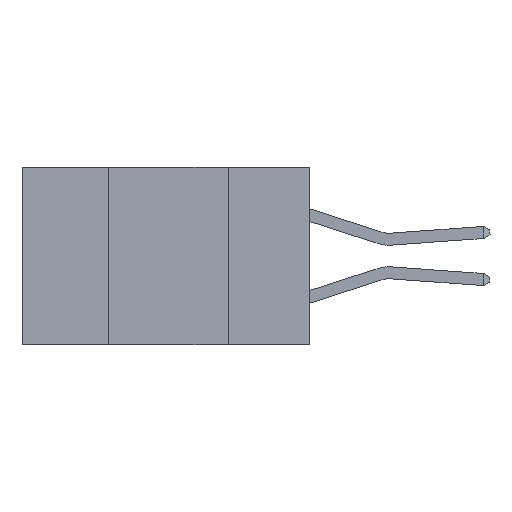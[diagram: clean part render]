
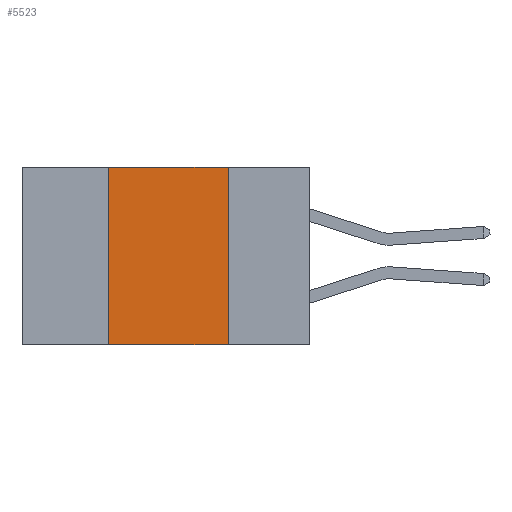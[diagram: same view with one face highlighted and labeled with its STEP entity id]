
A CAD part, left-side view. The second image highlights one B-rep face of the part: STEP entity #5523.
In plain terms, the highlighted planar face has unit normal (-1, 0, 0).
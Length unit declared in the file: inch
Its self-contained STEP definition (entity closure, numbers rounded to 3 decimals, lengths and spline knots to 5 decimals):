
#82 = FACE_OUTER_BOUND ( 'NONE', #3241, .T. ) ;
#1357 = ORIENTED_EDGE ( 'NONE', *, *, #4024, .F. ) ;
#2063 = CARTESIAN_POINT ( 'NONE',  ( 0., 0.6, -0.37 ) ) ;
#3241 = EDGE_LOOP ( 'NONE', ( #1357, #10445, #5084, #19178 ) ) ;
#3884 = DIRECTION ( 'NONE',  ( 0., -1., 0. ) ) ;
#4024 = EDGE_CURVE ( 'NONE', #11356, #23159, #18539, .T. ) ;
#4335 = LINE ( 'NONE', #2063, #17885 ) ;
#5084 = ORIENTED_EDGE ( 'NONE', *, *, #20491, .F. ) ;
#5523 = ADVANCED_FACE ( 'NONE', ( #82 ), #11019, .F. ) ;
#7018 = AXIS2_PLACEMENT_3D ( 'NONE', #10941, #9634, #9485 ) ;
#7191 = VERTEX_POINT ( 'NONE', #11721 ) ;
#8493 = CARTESIAN_POINT ( 'NONE',  ( 0., 0.17, -0.37 ) ) ;
#8688 = DIRECTION ( 'NONE',  ( 0., -1., 0. ) ) ;
#9030 = VECTOR ( 'NONE', #8688, 39.37008 ) ;
#9071 = VECTOR ( 'NONE', #11891, 39.37008 ) ;
#9485 = DIRECTION ( 'NONE',  ( 0., 0., -1. ) ) ;
#9634 = DIRECTION ( 'NONE',  ( 1., 0., 0. ) ) ;
#10445 = ORIENTED_EDGE ( 'NONE', *, *, #22033, .F. ) ;
#10941 = CARTESIAN_POINT ( 'NONE',  ( 0., 0.6, 0. ) ) ;
#11019 = PLANE ( 'NONE',  #7018 ) ;
#11356 = VERTEX_POINT ( 'NONE', #14112 ) ;
#11721 = CARTESIAN_POINT ( 'NONE',  ( 0., 0.42, 0. ) ) ;
#11891 = DIRECTION ( 'NONE',  ( 0., 0., 1. ) ) ;
#12679 = CARTESIAN_POINT ( 'NONE',  ( 0., 0.17, 0. ) ) ;
#12963 = VERTEX_POINT ( 'NONE', #16000 ) ;
#13809 = DIRECTION ( 'NONE',  ( 0., 0., -1. ) ) ;
#13973 = LINE ( 'NONE', #21556, #9030 ) ;
#14112 = CARTESIAN_POINT ( 'NONE',  ( 0., 0.17, 0. ) ) ;
#14613 = LINE ( 'NONE', #17500, #9071 ) ;
#16000 = CARTESIAN_POINT ( 'NONE',  ( 0., 0.42, -0.37 ) ) ;
#16835 = EDGE_CURVE ( 'NONE', #12963, #23159, #4335, .T. ) ;
#17500 = CARTESIAN_POINT ( 'NONE',  ( 0., 0.42, 0. ) ) ;
#17885 = VECTOR ( 'NONE', #3884, 39.37008 ) ;
#18539 = LINE ( 'NONE', #12679, #23362 ) ;
#19178 = ORIENTED_EDGE ( 'NONE', *, *, #16835, .T. ) ;
#20491 = EDGE_CURVE ( 'NONE', #12963, #7191, #14613, .T. ) ;
#21556 = CARTESIAN_POINT ( 'NONE',  ( 0., 0.6, 0. ) ) ;
#22033 = EDGE_CURVE ( 'NONE', #7191, #11356, #13973, .T. ) ;
#23159 = VERTEX_POINT ( 'NONE', #8493 ) ;
#23362 = VECTOR ( 'NONE', #13809, 39.37008 ) ;
